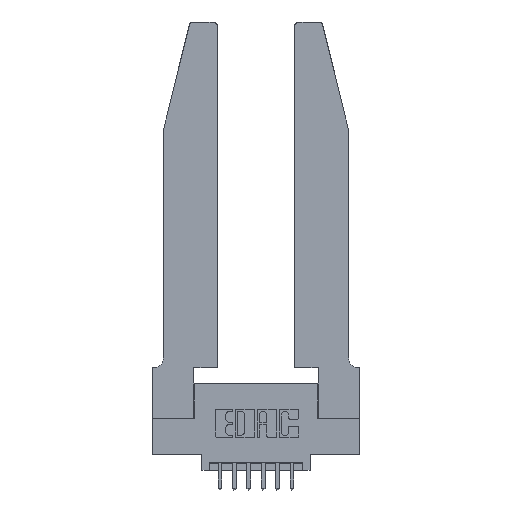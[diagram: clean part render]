
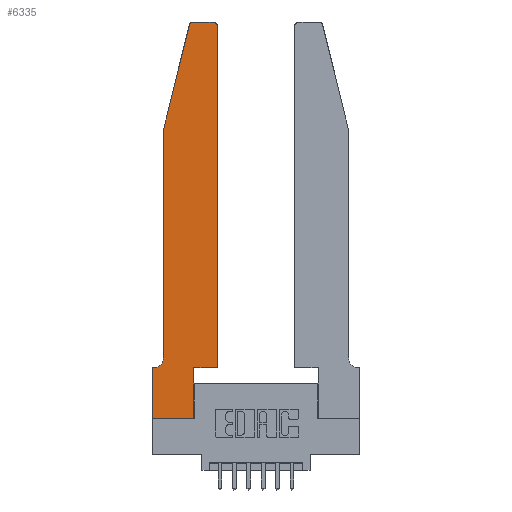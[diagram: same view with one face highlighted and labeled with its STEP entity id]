
A CAD part, top view. The second image highlights one B-rep face of the part: STEP entity #6335.
In plain terms, the highlighted planar face has unit normal (0, 0, 1).
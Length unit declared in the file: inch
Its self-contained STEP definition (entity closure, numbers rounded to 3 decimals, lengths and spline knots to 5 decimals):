
#177 = CARTESIAN_POINT ( 'NONE',  ( 0.4505, 0.35, 0.37 ) ) ;
#214 = CARTESIAN_POINT ( 'NONE',  ( 0.284, 2.75, 0.37 ) ) ;
#346 = VERTEX_POINT ( 'NONE', #214 ) ;
#756 = VECTOR ( 'NONE', #9903, 39.37008 ) ;
#781 = CARTESIAN_POINT ( 'NONE',  ( 0.2865, 0.35, 0.37 ) ) ;
#896 = VERTEX_POINT ( 'NONE', #984 ) ;
#909 = VECTOR ( 'NONE', #10913, 39.37008 ) ;
#984 = CARTESIAN_POINT ( 'NONE',  ( 0., 0.35, 0.37 ) ) ;
#1093 = EDGE_CURVE ( 'NONE', #346, #7600, #9754, .T. ) ;
#1149 = LINE ( 'NONE', #781, #5349 ) ;
#1332 = CARTESIAN_POINT ( 'NONE',  ( 0.4205, 2.75, 0.37 ) ) ;
#1667 = CIRCLE ( 'NONE', #4643, 0.07 ) ;
#1925 = LINE ( 'NONE', #8142, #10127 ) ;
#1929 = VECTOR ( 'NONE', #6497, 39.37008 ) ;
#2073 = CARTESIAN_POINT ( 'NONE',  ( 0.4505, 0.35, 0.37 ) ) ;
#2154 = DIRECTION ( 'NONE',  ( 0., -1., 0. ) ) ;
#2251 = CARTESIAN_POINT ( 'NONE',  ( 0.0755, 2., 0.37 ) ) ;
#2265 = ORIENTED_EDGE ( 'NONE', *, *, #7004, .T. ) ;
#2274 = ORIENTED_EDGE ( 'NONE', *, *, #1093, .T. ) ;
#2338 = CARTESIAN_POINT ( 'NONE',  ( 0.0755, 0.35, 0.37 ) ) ;
#2389 = ORIENTED_EDGE ( 'NONE', *, *, #13348, .T. ) ;
#2425 = DIRECTION ( 'NONE',  ( 0., 0., 1. ) ) ;
#2494 = ORIENTED_EDGE ( 'NONE', *, *, #5475, .T. ) ;
#2495 = LINE ( 'NONE', #11917, #14018 ) ;
#2658 = CARTESIAN_POINT ( 'NONE',  ( 0.2865, 0., 0.37 ) ) ;
#3110 = ORIENTED_EDGE ( 'NONE', *, *, #12275, .T. ) ;
#3364 = CARTESIAN_POINT ( 'NONE',  ( 0.4205, 2.72, 0.37 ) ) ;
#3867 = CARTESIAN_POINT ( 'NONE',  ( 0., 0., 0.37 ) ) ;
#3880 = PLANE ( 'NONE',  #3997 ) ;
#3911 = CARTESIAN_POINT ( 'NONE',  ( 0., 0., 0.37 ) ) ;
#3997 = AXIS2_PLACEMENT_3D ( 'NONE', #9571, #11680, #5001 ) ;
#4032 = AXIS2_PLACEMENT_3D ( 'NONE', #8060, #2425, #10125 ) ;
#4255 = DIRECTION ( 'NONE',  ( -0.239, -0.971, 0. ) ) ;
#4468 = EDGE_CURVE ( 'NONE', #12322, #7857, #1667, .T. ) ;
#4643 = AXIS2_PLACEMENT_3D ( 'NONE', #10416, #7126, #6103 ) ;
#4780 = VECTOR ( 'NONE', #12424, 39.37008 ) ;
#5001 = DIRECTION ( 'NONE',  ( 1., 0., 0. ) ) ;
#5349 = VECTOR ( 'NONE', #8646, 39.37008 ) ;
#5431 = CARTESIAN_POINT ( 'NONE',  ( 0.2605, 2.75, 0.37 ) ) ;
#5475 = EDGE_CURVE ( 'NONE', #7857, #896, #9310, .T. ) ;
#5498 = CARTESIAN_POINT ( 'NONE',  ( 0.0755, 2., 0.37 ) ) ;
#5567 = LINE ( 'NONE', #3867, #12691 ) ;
#5631 = EDGE_CURVE ( 'NONE', #7600, #11899, #2495, .T. ) ;
#5759 = CARTESIAN_POINT ( 'NONE',  ( 0.25487, 2.72718, 0.37 ) ) ;
#5793 = CARTESIAN_POINT ( 'NONE',  ( 0., 0., 0.37 ) ) ;
#5926 = ORIENTED_EDGE ( 'NONE', *, *, #5631, .T. ) ;
#6037 = EDGE_CURVE ( 'NONE', #896, #13550, #13288, .T. ) ;
#6103 = DIRECTION ( 'NONE',  ( -1., 0., 0. ) ) ;
#6269 = VERTEX_POINT ( 'NONE', #177 ) ;
#6335 = ADVANCED_FACE ( 'NONE', ( #10154 ), #3880, .T. ) ;
#6497 = DIRECTION ( 'NONE',  ( 1., 0., 0. ) ) ;
#6762 = CARTESIAN_POINT ( 'NONE',  ( 0.4505, 2.72, 0.37 ) ) ;
#7004 = EDGE_CURVE ( 'NONE', #12296, #6269, #11019, .T. ) ;
#7126 = DIRECTION ( 'NONE',  ( 0., 0., -1. ) ) ;
#7271 = LINE ( 'NONE', #5431, #756 ) ;
#7312 = ORIENTED_EDGE ( 'NONE', *, *, #10201, .T. ) ;
#7591 = AXIS2_PLACEMENT_3D ( 'NONE', #3364, #11185, #7694 ) ;
#7600 = VERTEX_POINT ( 'NONE', #5759 ) ;
#7694 = DIRECTION ( 'NONE',  ( 1., 0., 0. ) ) ;
#7750 = CARTESIAN_POINT ( 'NONE',  ( 0.2865, 0.35, 0.37 ) ) ;
#7857 = VERTEX_POINT ( 'NONE', #11937 ) ;
#8060 = CARTESIAN_POINT ( 'NONE',  ( 0.284, 2.72, 0.37 ) ) ;
#8142 = CARTESIAN_POINT ( 'NONE',  ( 0.4505, 0.35, 0.37 ) ) ;
#8195 = EDGE_CURVE ( 'NONE', #6269, #12346, #1925, .T. ) ;
#8646 = DIRECTION ( 'NONE',  ( 0., 1., 0. ) ) ;
#8854 = ORIENTED_EDGE ( 'NONE', *, *, #6037, .T. ) ;
#8873 = ORIENTED_EDGE ( 'NONE', *, *, #11671, .T. ) ;
#9243 = EDGE_LOOP ( 'NONE', ( #3110, #2274, #5926, #2389, #11233, #2494, #8854, #11432, #8873, #2265, #11410, #7312 ) ) ;
#9310 = LINE ( 'NONE', #2338, #4780 ) ;
#9367 = DIRECTION ( 'NONE',  ( 1., 0., 0. ) ) ;
#9508 = EDGE_CURVE ( 'NONE', #13550, #11474, #5567, .T. ) ;
#9571 = CARTESIAN_POINT ( 'NONE',  ( 0., 0.35, 0.37 ) ) ;
#9754 = CIRCLE ( 'NONE', #4032, 0.03 ) ;
#9903 = DIRECTION ( 'NONE',  ( -1., 0., 0. ) ) ;
#10125 = DIRECTION ( 'NONE',  ( 1., 0., 0. ) ) ;
#10127 = VECTOR ( 'NONE', #11674, 39.37008 ) ;
#10154 = FACE_OUTER_BOUND ( 'NONE', #9243, .T. ) ;
#10201 = EDGE_CURVE ( 'NONE', #12346, #11961, #10942, .T. ) ;
#10416 = CARTESIAN_POINT ( 'NONE',  ( 0.0055, 0.42, 0.37 ) ) ;
#10913 = DIRECTION ( 'NONE',  ( 0., -1., 0. ) ) ;
#10942 = CIRCLE ( 'NONE', #7591, 0.03 ) ;
#11019 = LINE ( 'NONE', #2073, #1929 ) ;
#11140 = CARTESIAN_POINT ( 'NONE',  ( 0.0755, 0.42, 0.37 ) ) ;
#11185 = DIRECTION ( 'NONE',  ( 0., 0., 1. ) ) ;
#11233 = ORIENTED_EDGE ( 'NONE', *, *, #4468, .T. ) ;
#11410 = ORIENTED_EDGE ( 'NONE', *, *, #8195, .T. ) ;
#11432 = ORIENTED_EDGE ( 'NONE', *, *, #9508, .T. ) ;
#11474 = VERTEX_POINT ( 'NONE', #2658 ) ;
#11671 = EDGE_CURVE ( 'NONE', #11474, #12296, #1149, .T. ) ;
#11674 = DIRECTION ( 'NONE',  ( 0., 1., 0. ) ) ;
#11680 = DIRECTION ( 'NONE',  ( 0., 0., 1. ) ) ;
#11899 = VERTEX_POINT ( 'NONE', #2251 ) ;
#11917 = CARTESIAN_POINT ( 'NONE',  ( 0.0755, 2., 0.37 ) ) ;
#11937 = CARTESIAN_POINT ( 'NONE',  ( 0.0055, 0.35, 0.37 ) ) ;
#11961 = VERTEX_POINT ( 'NONE', #1332 ) ;
#12275 = EDGE_CURVE ( 'NONE', #11961, #346, #7271, .T. ) ;
#12296 = VERTEX_POINT ( 'NONE', #7750 ) ;
#12322 = VERTEX_POINT ( 'NONE', #11140 ) ;
#12346 = VERTEX_POINT ( 'NONE', #6762 ) ;
#12424 = DIRECTION ( 'NONE',  ( -1., 0., 0. ) ) ;
#12691 = VECTOR ( 'NONE', #9367, 39.37008 ) ;
#13288 = LINE ( 'NONE', #3911, #909 ) ;
#13306 = LINE ( 'NONE', #5498, #13657 ) ;
#13348 = EDGE_CURVE ( 'NONE', #11899, #12322, #13306, .T. ) ;
#13550 = VERTEX_POINT ( 'NONE', #5793 ) ;
#13657 = VECTOR ( 'NONE', #2154, 39.37008 ) ;
#14018 = VECTOR ( 'NONE', #4255, 39.37008 ) ;
